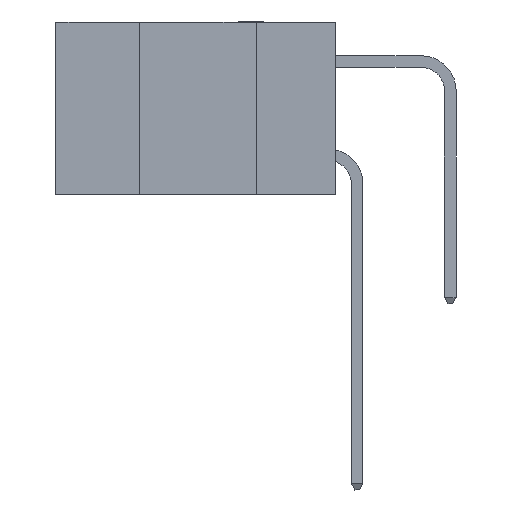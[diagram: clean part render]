
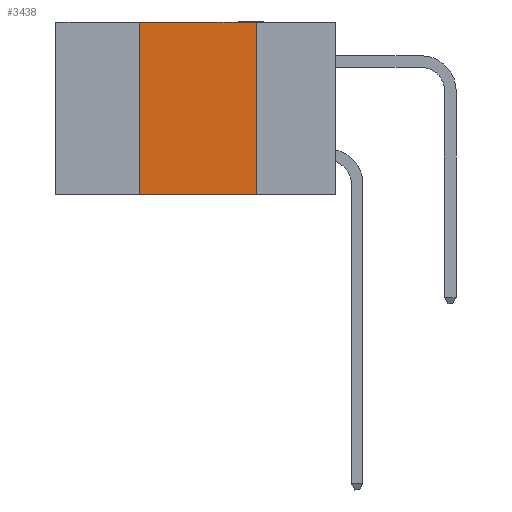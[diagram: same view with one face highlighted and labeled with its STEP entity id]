
A CAD part, left-side view. The second image highlights one B-rep face of the part: STEP entity #3438.
In plain terms, the highlighted planar face has unit normal (-1, 0, 0).
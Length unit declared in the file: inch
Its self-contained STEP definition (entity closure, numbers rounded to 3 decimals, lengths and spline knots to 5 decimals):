
#673 = ORIENTED_EDGE ( 'NONE', *, *, #8368, .F. ) ;
#1890 = CARTESIAN_POINT ( 'NONE',  ( 0., 0.17, -0.37 ) ) ;
#2015 = VERTEX_POINT ( 'NONE', #19602 ) ;
#3438 = ADVANCED_FACE ( 'NONE', ( #16057 ), #23781, .F. ) ;
#3745 = ORIENTED_EDGE ( 'NONE', *, *, #26160, .F. ) ;
#4464 = EDGE_LOOP ( 'NONE', ( #15390, #3745, #673, #15850 ) ) ;
#8252 = LINE ( 'NONE', #26105, #11209 ) ;
#8368 = EDGE_CURVE ( 'NONE', #2015, #15298, #28657, .T. ) ;
#9000 = DIRECTION ( 'NONE',  ( 0., 0., 1. ) ) ;
#9382 = CARTESIAN_POINT ( 'NONE',  ( 0., 0.42, 0. ) ) ;
#9438 = DIRECTION ( 'NONE',  ( 0., -1., 0. ) ) ;
#9907 = DIRECTION ( 'NONE',  ( 0., 0., -1. ) ) ;
#11209 = VECTOR ( 'NONE', #9438, 39.37008 ) ;
#14843 = LINE ( 'NONE', #29286, #22269 ) ;
#15298 = VERTEX_POINT ( 'NONE', #9382 ) ;
#15390 = ORIENTED_EDGE ( 'NONE', *, *, #15410, .F. ) ;
#15410 = EDGE_CURVE ( 'NONE', #26722, #16458, #17712, .T. ) ;
#15850 = ORIENTED_EDGE ( 'NONE', *, *, #24029, .T. ) ;
#16057 = FACE_OUTER_BOUND ( 'NONE', #4464, .T. ) ;
#16458 = VERTEX_POINT ( 'NONE', #1890 ) ;
#17712 = LINE ( 'NONE', #34574, #31288 ) ;
#18327 = DIRECTION ( 'NONE',  ( 1., 0., 0. ) ) ;
#19602 = CARTESIAN_POINT ( 'NONE',  ( 0., 0.42, -0.37 ) ) ;
#21049 = CARTESIAN_POINT ( 'NONE',  ( 0., 0.6, 0. ) ) ;
#21226 = VECTOR ( 'NONE', #9000, 39.37008 ) ;
#22269 = VECTOR ( 'NONE', #23597, 39.37008 ) ;
#23292 = AXIS2_PLACEMENT_3D ( 'NONE', #21049, #18327, #9907 ) ;
#23597 = DIRECTION ( 'NONE',  ( 0., -1., 0. ) ) ;
#23781 = PLANE ( 'NONE',  #23292 ) ;
#24029 = EDGE_CURVE ( 'NONE', #2015, #16458, #14843, .T. ) ;
#26105 = CARTESIAN_POINT ( 'NONE',  ( 0., 0.6, 0. ) ) ;
#26160 = EDGE_CURVE ( 'NONE', #15298, #26722, #8252, .T. ) ;
#26722 = VERTEX_POINT ( 'NONE', #31670 ) ;
#28657 = LINE ( 'NONE', #30389, #21226 ) ;
#29286 = CARTESIAN_POINT ( 'NONE',  ( 0., 0.6, -0.37 ) ) ;
#30389 = CARTESIAN_POINT ( 'NONE',  ( 0., 0.42, 0. ) ) ;
#31288 = VECTOR ( 'NONE', #34208, 39.37008 ) ;
#31670 = CARTESIAN_POINT ( 'NONE',  ( 0., 0.17, 0. ) ) ;
#34208 = DIRECTION ( 'NONE',  ( 0., 0., -1. ) ) ;
#34574 = CARTESIAN_POINT ( 'NONE',  ( 0., 0.17, 0. ) ) ;
